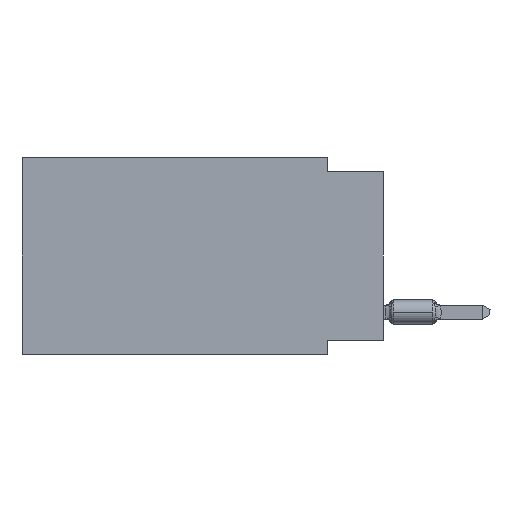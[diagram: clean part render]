
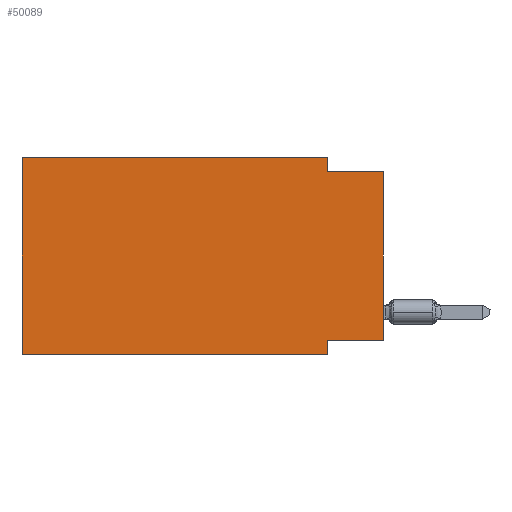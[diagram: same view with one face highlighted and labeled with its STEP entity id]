
A CAD part, left-side view. The second image highlights one B-rep face of the part: STEP entity #50089.
In plain terms, the highlighted planar face has unit normal (-1, 0, 0).
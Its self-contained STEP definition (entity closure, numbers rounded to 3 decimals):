
#734 = AXIS2_PLACEMENT_3D ( 'NONE', #4409, #47412, #12785 ) ;
#2391 = DIRECTION ( 'NONE',  ( 0., 0., -1. ) ) ;
#2680 = CARTESIAN_POINT ( 'NONE',  ( 0., 2.54, 0. ) ) ;
#4052 = ORIENTED_EDGE ( 'NONE', *, *, #8067, .F. ) ;
#4409 = CARTESIAN_POINT ( 'NONE',  ( 0., 16.383, 0. ) ) ;
#4928 = EDGE_CURVE ( 'NONE', #41687, #38239, #46490, .T. ) ;
#5767 = VECTOR ( 'NONE', #14697, 1000. ) ;
#7188 = CARTESIAN_POINT ( 'NONE',  ( 0., 16.383, 0. ) ) ;
#7657 = EDGE_CURVE ( 'NONE', #45430, #9517, #18068, .T. ) ;
#8067 = EDGE_CURVE ( 'NONE', #38239, #16104, #35421, .T. ) ;
#8251 = CARTESIAN_POINT ( 'NONE',  ( 0., 2.54, 0. ) ) ;
#8831 = CARTESIAN_POINT ( 'NONE',  ( 0., 0., -0.635 ) ) ;
#9517 = VERTEX_POINT ( 'NONE', #15928 ) ;
#10383 = EDGE_CURVE ( 'NONE', #51679, #9517, #27260, .T. ) ;
#10386 = EDGE_CURVE ( 'NONE', #51994, #16104, #36732, .T. ) ;
#10798 = LINE ( 'NONE', #27824, #19772 ) ;
#11668 = VECTOR ( 'NONE', #21072, 1000. ) ;
#12785 = DIRECTION ( 'NONE',  ( 0., 0., -1. ) ) ;
#14697 = DIRECTION ( 'NONE',  ( 0., -1., 0. ) ) ;
#14739 = VECTOR ( 'NONE', #48276, 1000. ) ;
#15928 = CARTESIAN_POINT ( 'NONE',  ( 0., 2.54, -8.89 ) ) ;
#16072 = CARTESIAN_POINT ( 'NONE',  ( 0., 0., -8.255 ) ) ;
#16104 = VERTEX_POINT ( 'NONE', #8831 ) ;
#18068 = LINE ( 'NONE', #31728, #5767 ) ;
#18348 = DIRECTION ( 'NONE',  ( 0., 1., 0. ) ) ;
#19232 = CARTESIAN_POINT ( 'NONE',  ( 0., 0., -0.635 ) ) ;
#19473 = ORIENTED_EDGE ( 'NONE', *, *, #46617, .F. ) ;
#19772 = VECTOR ( 'NONE', #18348, 1000. ) ;
#19957 = EDGE_CURVE ( 'NONE', #45430, #28842, #52143, .T. ) ;
#19985 = CARTESIAN_POINT ( 'NONE',  ( 0., 2.54, -8.89 ) ) ;
#21072 = DIRECTION ( 'NONE',  ( 0., 0., -1. ) ) ;
#24540 = VECTOR ( 'NONE', #2391, 1000. ) ;
#25561 = EDGE_CURVE ( 'NONE', #51994, #51679, #10798, .T. ) ;
#27260 = LINE ( 'NONE', #19985, #24540 ) ;
#27816 = CARTESIAN_POINT ( 'NONE',  ( 0., 0., 0. ) ) ;
#27824 = CARTESIAN_POINT ( 'NONE',  ( 0., 0., -8.255 ) ) ;
#28463 = CARTESIAN_POINT ( 'NONE',  ( 0., 16.383, -8.89 ) ) ;
#28842 = VERTEX_POINT ( 'NONE', #39537 ) ;
#28880 = ORIENTED_EDGE ( 'NONE', *, *, #10383, .F. ) ;
#29136 = VECTOR ( 'NONE', #29833, 1000. ) ;
#29833 = DIRECTION ( 'NONE',  ( 0., 0., 1. ) ) ;
#31728 = CARTESIAN_POINT ( 'NONE',  ( 0., 16.383, -8.89 ) ) ;
#34336 = VECTOR ( 'NONE', #53768, 1000. ) ;
#35355 = CARTESIAN_POINT ( 'NONE',  ( 0., 2.54, -8.255 ) ) ;
#35421 = LINE ( 'NONE', #19232, #14739 ) ;
#35884 = ORIENTED_EDGE ( 'NONE', *, *, #19957, .F. ) ;
#36732 = LINE ( 'NONE', #27816, #34336 ) ;
#36766 = LINE ( 'NONE', #7188, #45409 ) ;
#38239 = VERTEX_POINT ( 'NONE', #51827 ) ;
#38472 = PLANE ( 'NONE',  #734 ) ;
#39537 = CARTESIAN_POINT ( 'NONE',  ( 0., 16.383, 0. ) ) ;
#41242 = ORIENTED_EDGE ( 'NONE', *, *, #7657, .T. ) ;
#41687 = VERTEX_POINT ( 'NONE', #2680 ) ;
#43629 = ORIENTED_EDGE ( 'NONE', *, *, #4928, .F. ) ;
#44356 = ORIENTED_EDGE ( 'NONE', *, *, #10386, .T. ) ;
#45409 = VECTOR ( 'NONE', #49895, 1000. ) ;
#45430 = VERTEX_POINT ( 'NONE', #28463 ) ;
#46490 = LINE ( 'NONE', #8251, #11668 ) ;
#46617 = EDGE_CURVE ( 'NONE', #28842, #41687, #36766, .T. ) ;
#47128 = FACE_OUTER_BOUND ( 'NONE', #53274, .T. ) ;
#47412 = DIRECTION ( 'NONE',  ( 1., 0., 0. ) ) ;
#48276 = DIRECTION ( 'NONE',  ( 0., -1., 0. ) ) ;
#49895 = DIRECTION ( 'NONE',  ( 0., -1., 0. ) ) ;
#50089 = ADVANCED_FACE ( 'NONE', ( #47128 ), #38472, .F. ) ;
#51039 = CARTESIAN_POINT ( 'NONE',  ( 0., 16.383, 0. ) ) ;
#51679 = VERTEX_POINT ( 'NONE', #35355 ) ;
#51827 = CARTESIAN_POINT ( 'NONE',  ( 0., 2.54, -0.635 ) ) ;
#51994 = VERTEX_POINT ( 'NONE', #16072 ) ;
#52048 = ORIENTED_EDGE ( 'NONE', *, *, #25561, .F. ) ;
#52143 = LINE ( 'NONE', #51039, #29136 ) ;
#53274 = EDGE_LOOP ( 'NONE', ( #44356, #4052, #43629, #19473, #35884, #41242, #28880, #52048 ) ) ;
#53768 = DIRECTION ( 'NONE',  ( 0., 0., 1. ) ) ;
